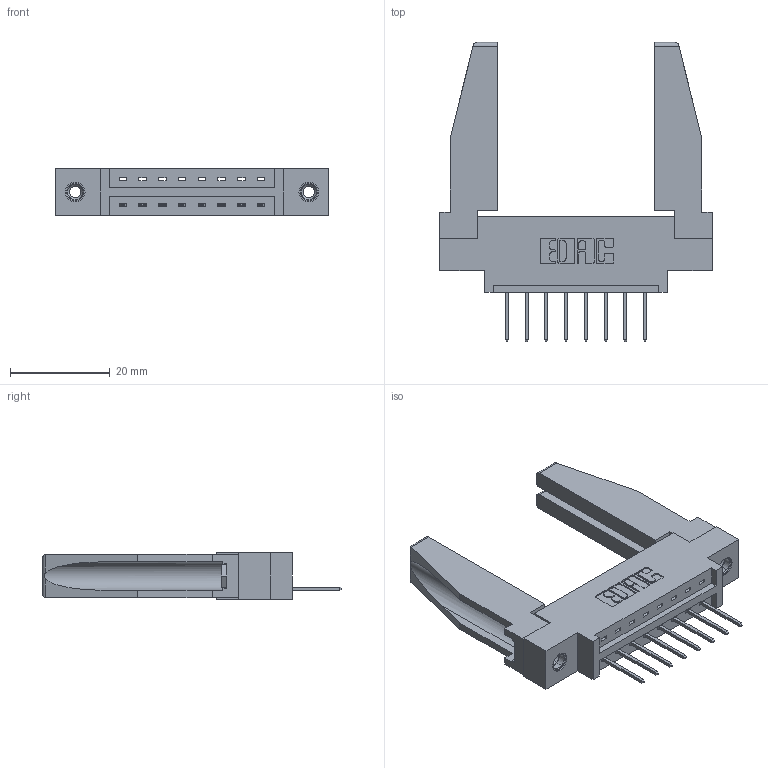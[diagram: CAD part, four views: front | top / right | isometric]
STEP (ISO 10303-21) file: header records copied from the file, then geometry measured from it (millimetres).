
FILE_DESCRIPTION (( 'STEP AP203' ), '1' );
FILE_NAME ('337-008-523-678.STEP', '2019-09-27T18:53:17', ( '' ), ( '' ), 'SwSTEP 2.0', 'SolidWorks 2016', '' );
FILE_SCHEMA (( 'CONFIG_CONTROL_DESIGN' ));
Length unit declared in the file: inch
Products named in the file (5): 337-008-523-678; 337 Part_0.170 Offset - 0.156 Dia-TI; 345-250-001_345-250-001-102; 345-292-001_345-293-123; 307-220-078
Assembly tree (13 placements, depth 2):
  337-008-523-678
    337 Part_0.170 Offset - 0.156 Dia-TI
    345-292-001_345-293-123  x8
    345-250-001_345-250-001-102  x2
    307-220-078  x2
Bounding box: 54.71 x 59.95 x 9.4 mm (x, y, z)
Volume: 9133.6 mm3; surface area: 9063.4 mm2
Topology: 13 solids, 13 shells, 744 faces, 2157 edges, 1418 vertices
Faces by surface type: plane 526, cylinder 202, cone 12, torus 4
Entity records: 12934 total; most frequent: CARTESIAN_POINT 2244, ORIENTED_EDGE 2144, DIRECTION 1968, EDGE_CURVE 1072, VECTOR 906, LINE 906, VERTEX_POINT 708, AXIS2_PLACEMENT_3D 531
